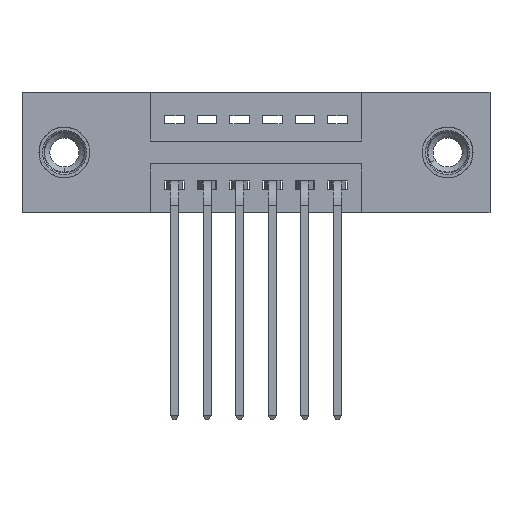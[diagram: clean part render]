
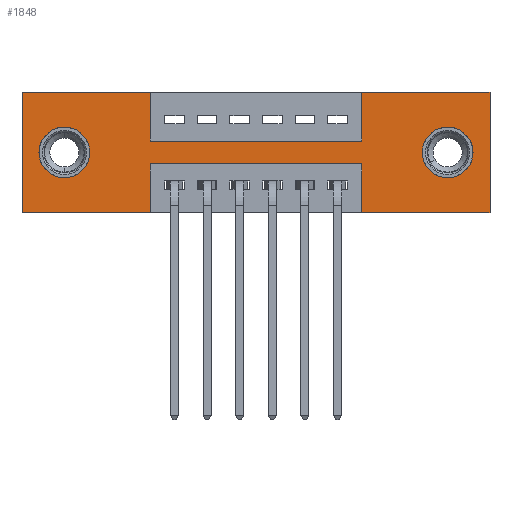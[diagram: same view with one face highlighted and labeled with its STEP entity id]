
A CAD part, front view. The second image highlights one B-rep face of the part: STEP entity #1848.
In plain terms, the highlighted planar face has unit normal (0, -1, 0).
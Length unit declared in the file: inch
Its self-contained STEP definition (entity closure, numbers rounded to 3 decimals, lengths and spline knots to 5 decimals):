
#185 = DIRECTION ( 'NONE',  ( 0., 0., 1. ) ) ;
#221 = CARTESIAN_POINT ( 'NONE',  ( 1.0425, 0., -0.37 ) ) ;
#269 = DIRECTION ( 'NONE',  ( 0., 0., 1. ) ) ;
#335 = DIRECTION ( 'NONE',  ( 0., 1., 0. ) ) ;
#369 = EDGE_CURVE ( 'NONE', #1914, #5391, #8173, .T. ) ;
#386 = EDGE_CURVE ( 'NONE', #5391, #5139, #8816, .T. ) ;
#438 = EDGE_LOOP ( 'NONE', ( #9791, #3066, #4372, #6042, #2475, #4582, #9256, #7584, #7389, #3813, #3783, #5017 ) ) ;
#514 = ORIENTED_EDGE ( 'NONE', *, *, #2277, .T. ) ;
#534 = VECTOR ( 'NONE', #10208, 39.37008 ) ;
#602 = VECTOR ( 'NONE', #10209, 39.37008 ) ;
#655 = DIRECTION ( 'NONE',  ( 0., 0., 1. ) ) ;
#662 = CARTESIAN_POINT ( 'NONE',  ( 0.3925, 0., 0. ) ) ;
#680 = CARTESIAN_POINT ( 'NONE',  ( 1.0425, 0., 0. ) ) ;
#902 = VERTEX_POINT ( 'NONE', #3952 ) ;
#1147 = LINE ( 'NONE', #221, #5295 ) ;
#1261 = CARTESIAN_POINT ( 'NONE',  ( 0.13, 0., -0.263 ) ) ;
#1293 = CARTESIAN_POINT ( 'NONE',  ( 1.0425, 0., -0.15 ) ) ;
#1310 = CARTESIAN_POINT ( 'NONE',  ( 0.3925, 0., -0.22 ) ) ;
#1460 = LINE ( 'NONE', #8265, #3270 ) ;
#1597 = AXIS2_PLACEMENT_3D ( 'NONE', #10558, #2265, #10413 ) ;
#1826 = CARTESIAN_POINT ( 'NONE',  ( 0., 0., 0. ) ) ;
#1848 = ADVANCED_FACE ( 'NONE', ( #10648, #3191, #4891 ), #7234, .T. ) ;
#1853 = VERTEX_POINT ( 'NONE', #3035 ) ;
#1914 = VERTEX_POINT ( 'NONE', #3326 ) ;
#1943 = EDGE_CURVE ( 'NONE', #7197, #7281, #10623, .T. ) ;
#1991 = DIRECTION ( 'NONE',  ( 0., 0., -1. ) ) ;
#2025 = EDGE_LOOP ( 'NONE', ( #7601, #6201 ) ) ;
#2064 = EDGE_CURVE ( 'NONE', #7211, #6184, #7132, .T. ) ;
#2098 = VERTEX_POINT ( 'NONE', #7897 ) ;
#2160 = VECTOR ( 'NONE', #3955, 39.37008 ) ;
#2183 = DIRECTION ( 'NONE',  ( -1., 0., 0. ) ) ;
#2208 = VERTEX_POINT ( 'NONE', #1826 ) ;
#2265 = DIRECTION ( 'NONE',  ( 0., -1., 0. ) ) ;
#2277 = EDGE_CURVE ( 'NONE', #3359, #9609, #3905, .T. ) ;
#2398 = CARTESIAN_POINT ( 'NONE',  ( 1.305, 0., -0.107 ) ) ;
#2402 = CARTESIAN_POINT ( 'NONE',  ( 0.13, 0., -0.185 ) ) ;
#2475 = ORIENTED_EDGE ( 'NONE', *, *, #7832, .F. ) ;
#2833 = LINE ( 'NONE', #10291, #3219 ) ;
#2855 = AXIS2_PLACEMENT_3D ( 'NONE', #2402, #3257, #8229 ) ;
#3035 = CARTESIAN_POINT ( 'NONE',  ( 1.435, 0., 0. ) ) ;
#3066 = ORIENTED_EDGE ( 'NONE', *, *, #2064, .F. ) ;
#3191 = FACE_BOUND ( 'NONE', #2025, .T. ) ;
#3219 = VECTOR ( 'NONE', #8761, 39.37008 ) ;
#3257 = DIRECTION ( 'NONE',  ( 0., 1., 0. ) ) ;
#3270 = VECTOR ( 'NONE', #6771, 39.37008 ) ;
#3326 = CARTESIAN_POINT ( 'NONE',  ( 0.3925, 0., 0. ) ) ;
#3359 = VERTEX_POINT ( 'NONE', #2398 ) ;
#3388 = EDGE_CURVE ( 'NONE', #902, #1853, #1460, .T. ) ;
#3421 = LINE ( 'NONE', #680, #6922 ) ;
#3504 = CARTESIAN_POINT ( 'NONE',  ( 0.3925, 0., -0.22 ) ) ;
#3518 = CARTESIAN_POINT ( 'NONE',  ( 0.3925, 0., -0.15 ) ) ;
#3624 = CARTESIAN_POINT ( 'NONE',  ( 1.435, 0., -0.37 ) ) ;
#3747 = EDGE_CURVE ( 'NONE', #4926, #4857, #4814, .T. ) ;
#3783 = ORIENTED_EDGE ( 'NONE', *, *, #4225, .F. ) ;
#3813 = ORIENTED_EDGE ( 'NONE', *, *, #6897, .F. ) ;
#3825 = CIRCLE ( 'NONE', #5071, 0.078 ) ;
#3856 = CIRCLE ( 'NONE', #9323, 0.078 ) ;
#3898 = CARTESIAN_POINT ( 'NONE',  ( 0.13, 0., -0.107 ) ) ;
#3905 = CIRCLE ( 'NONE', #8179, 0.078 ) ;
#3952 = CARTESIAN_POINT ( 'NONE',  ( 1.0425, 0., 0. ) ) ;
#3955 = DIRECTION ( 'NONE',  ( 0., 0., -1. ) ) ;
#4203 = CARTESIAN_POINT ( 'NONE',  ( 0., 0., -0.37 ) ) ;
#4225 = EDGE_CURVE ( 'NONE', #2098, #2208, #10489, .T. ) ;
#4372 = ORIENTED_EDGE ( 'NONE', *, *, #7557, .F. ) ;
#4472 = CARTESIAN_POINT ( 'NONE',  ( 0., 0., 0. ) ) ;
#4512 = CARTESIAN_POINT ( 'NONE',  ( 0., 0., -0.37 ) ) ;
#4582 = ORIENTED_EDGE ( 'NONE', *, *, #3388, .F. ) ;
#4804 = CARTESIAN_POINT ( 'NONE',  ( 1.305, 0., -0.263 ) ) ;
#4814 = LINE ( 'NONE', #4512, #602 ) ;
#4857 = VERTEX_POINT ( 'NONE', #10125 ) ;
#4891 = FACE_OUTER_BOUND ( 'NONE', #438, .T. ) ;
#4926 = VERTEX_POINT ( 'NONE', #3624 ) ;
#5017 = ORIENTED_EDGE ( 'NONE', *, *, #7045, .F. ) ;
#5071 = AXIS2_PLACEMENT_3D ( 'NONE', #7765, #335, #269 ) ;
#5139 = VERTEX_POINT ( 'NONE', #1293 ) ;
#5295 = VECTOR ( 'NONE', #185, 39.37008 ) ;
#5391 = VERTEX_POINT ( 'NONE', #3518 ) ;
#5429 = CARTESIAN_POINT ( 'NONE',  ( 0., 0., 0. ) ) ;
#5657 = ORIENTED_EDGE ( 'NONE', *, *, #10395, .T. ) ;
#5791 = DIRECTION ( 'NONE',  ( -1., 0., 0. ) ) ;
#6032 = DIRECTION ( 'NONE',  ( 0., 0., -1. ) ) ;
#6042 = ORIENTED_EDGE ( 'NONE', *, *, #3747, .F. ) ;
#6184 = VERTEX_POINT ( 'NONE', #3504 ) ;
#6201 = ORIENTED_EDGE ( 'NONE', *, *, #1943, .T. ) ;
#6528 = VECTOR ( 'NONE', #10364, 39.37008 ) ;
#6633 = VECTOR ( 'NONE', #2183, 39.37008 ) ;
#6743 = CARTESIAN_POINT ( 'NONE',  ( 1.305, 0., -0.185 ) ) ;
#6771 = DIRECTION ( 'NONE',  ( 1., 0., 0. ) ) ;
#6897 = EDGE_CURVE ( 'NONE', #2208, #1914, #7114, .T. ) ;
#6922 = VECTOR ( 'NONE', #655, 39.37008 ) ;
#6955 = CARTESIAN_POINT ( 'NONE',  ( 1.305, 0., -0.185 ) ) ;
#7021 = VECTOR ( 'NONE', #7248, 39.37008 ) ;
#7045 = EDGE_CURVE ( 'NONE', #7357, #2098, #7238, .T. ) ;
#7110 = EDGE_CURVE ( 'NONE', #6184, #7357, #2833, .T. ) ;
#7114 = LINE ( 'NONE', #4472, #534 ) ;
#7132 = LINE ( 'NONE', #1310, #6633 ) ;
#7197 = VERTEX_POINT ( 'NONE', #1261 ) ;
#7211 = VERTEX_POINT ( 'NONE', #9605 ) ;
#7234 = PLANE ( 'NONE',  #1597 ) ;
#7238 = LINE ( 'NONE', #4203, #7617 ) ;
#7248 = DIRECTION ( 'NONE',  ( 0., 0., -1. ) ) ;
#7281 = VERTEX_POINT ( 'NONE', #3898 ) ;
#7357 = VERTEX_POINT ( 'NONE', #10497 ) ;
#7389 = ORIENTED_EDGE ( 'NONE', *, *, #369, .F. ) ;
#7557 = EDGE_CURVE ( 'NONE', #4857, #7211, #1147, .T. ) ;
#7584 = ORIENTED_EDGE ( 'NONE', *, *, #386, .F. ) ;
#7601 = ORIENTED_EDGE ( 'NONE', *, *, #9961, .T. ) ;
#7617 = VECTOR ( 'NONE', #5791, 39.37008 ) ;
#7765 = CARTESIAN_POINT ( 'NONE',  ( 0.13, 0., -0.185 ) ) ;
#7779 = EDGE_LOOP ( 'NONE', ( #514, #5657 ) ) ;
#7832 = EDGE_CURVE ( 'NONE', #1853, #4926, #9016, .T. ) ;
#7897 = CARTESIAN_POINT ( 'NONE',  ( 0., 0., -0.37 ) ) ;
#7968 = CARTESIAN_POINT ( 'NONE',  ( 1.435, 0., 0. ) ) ;
#8173 = LINE ( 'NONE', #662, #7021 ) ;
#8179 = AXIS2_PLACEMENT_3D ( 'NONE', #6743, #9225, #1991 ) ;
#8229 = DIRECTION ( 'NONE',  ( 0., 0., 1. ) ) ;
#8265 = CARTESIAN_POINT ( 'NONE',  ( 0., 0., 0. ) ) ;
#8454 = DIRECTION ( 'NONE',  ( 0., 1., 0. ) ) ;
#8761 = DIRECTION ( 'NONE',  ( 0., 0., -1. ) ) ;
#8816 = LINE ( 'NONE', #9759, #10482 ) ;
#9016 = LINE ( 'NONE', #7968, #2160 ) ;
#9225 = DIRECTION ( 'NONE',  ( 0., 1., 0. ) ) ;
#9256 = ORIENTED_EDGE ( 'NONE', *, *, #9581, .F. ) ;
#9323 = AXIS2_PLACEMENT_3D ( 'NONE', #6955, #8454, #6032 ) ;
#9581 = EDGE_CURVE ( 'NONE', #5139, #902, #3421, .T. ) ;
#9605 = CARTESIAN_POINT ( 'NONE',  ( 1.0425, 0., -0.22 ) ) ;
#9609 = VERTEX_POINT ( 'NONE', #4804 ) ;
#9759 = CARTESIAN_POINT ( 'NONE',  ( 0.3925, 0., -0.15 ) ) ;
#9791 = ORIENTED_EDGE ( 'NONE', *, *, #7110, .F. ) ;
#9961 = EDGE_CURVE ( 'NONE', #7281, #7197, #3825, .T. ) ;
#10125 = CARTESIAN_POINT ( 'NONE',  ( 1.0425, 0., -0.37 ) ) ;
#10208 = DIRECTION ( 'NONE',  ( 1., 0., 0. ) ) ;
#10209 = DIRECTION ( 'NONE',  ( -1., 0., 0. ) ) ;
#10291 = CARTESIAN_POINT ( 'NONE',  ( 0.3925, 0., -0.37 ) ) ;
#10364 = DIRECTION ( 'NONE',  ( 0., 0., 1. ) ) ;
#10395 = EDGE_CURVE ( 'NONE', #9609, #3359, #3856, .T. ) ;
#10413 = DIRECTION ( 'NONE',  ( 0., 0., -1. ) ) ;
#10482 = VECTOR ( 'NONE', #10511, 39.37008 ) ;
#10489 = LINE ( 'NONE', #5429, #6528 ) ;
#10497 = CARTESIAN_POINT ( 'NONE',  ( 0.3925, 0., -0.37 ) ) ;
#10511 = DIRECTION ( 'NONE',  ( 1., 0., 0. ) ) ;
#10558 = CARTESIAN_POINT ( 'NONE',  ( 0., 0., -0.37 ) ) ;
#10623 = CIRCLE ( 'NONE', #2855, 0.078 ) ;
#10648 = FACE_BOUND ( 'NONE', #7779, .T. ) ;
